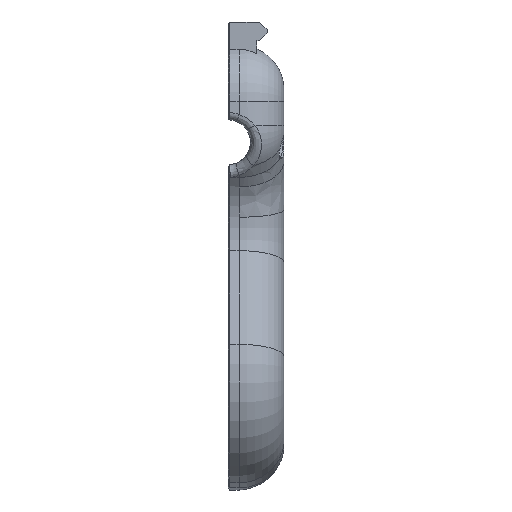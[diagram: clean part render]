
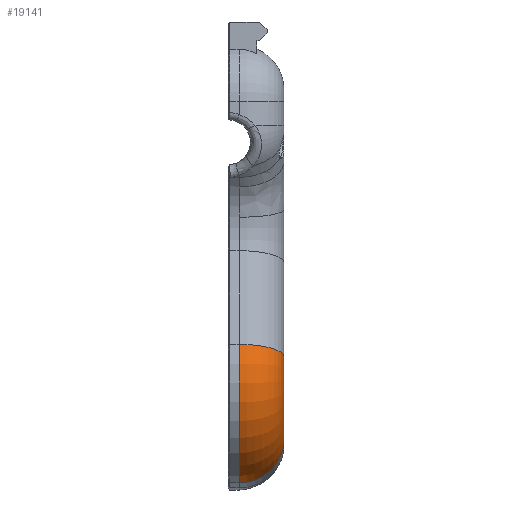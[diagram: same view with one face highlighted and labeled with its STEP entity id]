
A CAD part, left-side view. The second image highlights one B-rep face of the part: STEP entity #19141.
In plain terms, the highlighted toroidal (fillet/blend) face has major radius 18 mm and minor radius 12 mm.
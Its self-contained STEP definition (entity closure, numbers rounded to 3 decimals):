
#64 = PLANE('',#65);
#65 = AXIS2_PLACEMENT_3D('',#66,#67,#68);
#66 = CARTESIAN_POINT('',(10.936,-15.,-32.273));
#67 = DIRECTION('',(0.,-1.,0.));
#68 = DIRECTION('',(0.,0.,-1.));
#674 = VERTEX_POINT('',#675);
#675 = CARTESIAN_POINT('',(-43.196,-15.,-74.47));
#689 = CYLINDRICAL_SURFACE('',#690,12.);
#690 = AXIS2_PLACEMENT_3D('',#691,#692,#693);
#691 = CARTESIAN_POINT('',(-43.196,-3.,-74.47));
#692 = DIRECTION('',(0.276,0.,0.961));
#693 = DIRECTION('',(0.,-1.,0.));
#701 = EDGE_CURVE('',#702,#674,#704,.T.);
#702 = VERTEX_POINT('',#703);
#703 = CARTESIAN_POINT('',(-30.855,-15.,-96.734));
#704 = SURFACE_CURVE('',#705,(#710,#721),.PCURVE_S1.);
#705 = CIRCLE('',#706,18.);
#706 = AXIS2_PLACEMENT_3D('',#707,#708,#709);
#707 = CARTESIAN_POINT('',(-25.893,-15.,-79.431));
#708 = DIRECTION('',(0.,1.,0.));
#709 = DIRECTION('',(-0.276,0.,-0.961));
#710 = PCURVE('',#64,#711);
#711 = DEFINITIONAL_REPRESENTATION('',(#712),#720);
#712 = ( BOUNDED_CURVE() B_SPLINE_CURVE(2,(#713,#714,#715,#716,#717,#718
,#719),.UNSPECIFIED.,.T.,.F.) B_SPLINE_CURVE_WITH_KNOTS((1,2,2,2,2,1),(
    -2.094,0.,2.094,4.189,6.283,
8.378),.UNSPECIFIED.) CURVE() GEOMETRIC_REPRESENTATION_ITEM() 
RATIONAL_B_SPLINE_CURVE((1.,0.5,1.,0.5,1.,0.5,1.)) REPRESENTATION_ITEM(
  '') );
#713 = CARTESIAN_POINT('',(64.461,-41.79));
#714 = CARTESIAN_POINT('',(55.867,-71.759));
#715 = CARTESIAN_POINT('',(34.21,-49.332));
#716 = CARTESIAN_POINT('',(12.553,-26.906));
#717 = CARTESIAN_POINT('',(42.803,-19.363));
#718 = CARTESIAN_POINT('',(73.054,-11.821));
#719 = CARTESIAN_POINT('',(64.461,-41.79));
#720 = ( GEOMETRIC_REPRESENTATION_CONTEXT(2) 
PARAMETRIC_REPRESENTATION_CONTEXT() REPRESENTATION_CONTEXT('2D SPACE',''
  ) );
#721 = PCURVE('',#722,#727);
#722 = TOROIDAL_SURFACE('',#723,18.,12.);
#723 = AXIS2_PLACEMENT_3D('',#724,#725,#726);
#724 = CARTESIAN_POINT('',(-25.893,-3.,-79.431));
#725 = DIRECTION('',(0.,1.,0.));
#726 = DIRECTION('',(-0.276,0.,-0.961));
#727 = DEFINITIONAL_REPRESENTATION('',(#728),#732);
#728 = LINE('',#729,#730);
#729 = CARTESIAN_POINT('',(0.,4.712));
#730 = VECTOR('',#731,1.);
#731 = DIRECTION('',(1.,0.));
#732 = ( GEOMETRIC_REPRESENTATION_CONTEXT(2) 
PARAMETRIC_REPRESENTATION_CONTEXT() REPRESENTATION_CONTEXT('2D SPACE',''
  ) );
#750 = CYLINDRICAL_SURFACE('',#751,12.);
#751 = AXIS2_PLACEMENT_3D('',#752,#753,#754);
#752 = CARTESIAN_POINT('',(-26.048,-3.,-98.112));
#753 = DIRECTION('',(-0.961,0.,0.276));
#754 = DIRECTION('',(0.,-1.,0.));
#19036 = VERTEX_POINT('',#19037);
#19037 = CARTESIAN_POINT('',(-34.162,-3.,-108.269));
#19063 = EDGE_CURVE('',#702,#19036,#19064,.T.);
#19064 = SURFACE_CURVE('',#19065,(#19070,#19076),.PCURVE_S1.);
#19065 = CIRCLE('',#19066,12.);
#19066 = AXIS2_PLACEMENT_3D('',#19067,#19068,#19069);
#19067 = CARTESIAN_POINT('',(-30.855,-3.,-96.734));
#19068 = DIRECTION('',(0.961,0.,-0.276));
#19069 = DIRECTION('',(0.,-1.,0.));
#19070 = PCURVE('',#750,#19071);
#19071 = DEFINITIONAL_REPRESENTATION('',(#19072),#19075);
#19072 = B_SPLINE_CURVE_WITH_KNOTS('',1,(#19073,#19074),.UNSPECIFIED.,
  .F.,.F.,(2,2),(0.,1.571),.PIECEWISE_BEZIER_KNOTS.);
#19073 = CARTESIAN_POINT('',(0.,5.));
#19074 = CARTESIAN_POINT('',(-1.571,5.));
#19075 = ( GEOMETRIC_REPRESENTATION_CONTEXT(2) 
PARAMETRIC_REPRESENTATION_CONTEXT() REPRESENTATION_CONTEXT('2D SPACE',''
  ) );
#19076 = PCURVE('',#722,#19077);
#19077 = DEFINITIONAL_REPRESENTATION('',(#19078),#19081);
#19078 = B_SPLINE_CURVE_WITH_KNOTS('',1,(#19079,#19080),.UNSPECIFIED.,
  .F.,.F.,(2,2),(0.,1.571),.PIECEWISE_BEZIER_KNOTS.);
#19079 = CARTESIAN_POINT('',(0.,4.712));
#19080 = CARTESIAN_POINT('',(0.,6.283));
#19081 = ( GEOMETRIC_REPRESENTATION_CONTEXT(2) 
PARAMETRIC_REPRESENTATION_CONTEXT() REPRESENTATION_CONTEXT('2D SPACE',''
  ) );
#19141 = ADVANCED_FACE('',(#19142),#722,.T.);
#19142 = FACE_BOUND('',#19143,.T.);
#19143 = EDGE_LOOP('',(#19144,#19145,#19146,#19168));
#19144 = ORIENTED_EDGE('',*,*,#19063,.F.);
#19145 = ORIENTED_EDGE('',*,*,#701,.T.);
#19146 = ORIENTED_EDGE('',*,*,#19147,.T.);
#19147 = EDGE_CURVE('',#674,#19148,#19150,.T.);
#19148 = VERTEX_POINT('',#19149);
#19149 = CARTESIAN_POINT('',(-54.731,-3.,-71.162));
#19150 = SURFACE_CURVE('',#19151,(#19156,#19162),.PCURVE_S1.);
#19151 = CIRCLE('',#19152,12.);
#19152 = AXIS2_PLACEMENT_3D('',#19153,#19154,#19155);
#19153 = CARTESIAN_POINT('',(-43.196,-3.,-74.47));
#19154 = DIRECTION('',(-0.276,0.,-0.961));
#19155 = DIRECTION('',(-0.961,0.,0.276));
#19156 = PCURVE('',#722,#19157);
#19157 = DEFINITIONAL_REPRESENTATION('',(#19158),#19161);
#19158 = B_SPLINE_CURVE_WITH_KNOTS('',1,(#19159,#19160),.UNSPECIFIED.,
  .F.,.F.,(2,2),(4.712,6.283),
  .PIECEWISE_BEZIER_KNOTS.);
#19159 = CARTESIAN_POINT('',(1.571,4.712));
#19160 = CARTESIAN_POINT('',(1.571,6.283));
#19161 = ( GEOMETRIC_REPRESENTATION_CONTEXT(2) 
PARAMETRIC_REPRESENTATION_CONTEXT() REPRESENTATION_CONTEXT('2D SPACE',''
  ) );
#19162 = PCURVE('',#689,#19163);
#19163 = DEFINITIONAL_REPRESENTATION('',(#19164),#19167);
#19164 = B_SPLINE_CURVE_WITH_KNOTS('',1,(#19165,#19166),.UNSPECIFIED.,
  .F.,.F.,(2,2),(4.712,6.283),
  .PIECEWISE_BEZIER_KNOTS.);
#19165 = CARTESIAN_POINT('',(0.,0.));
#19166 = CARTESIAN_POINT('',(-1.571,0.));
#19167 = ( GEOMETRIC_REPRESENTATION_CONTEXT(2) 
PARAMETRIC_REPRESENTATION_CONTEXT() REPRESENTATION_CONTEXT('2D SPACE',''
  ) );
#19168 = ORIENTED_EDGE('',*,*,#19169,.F.);
#19169 = EDGE_CURVE('',#19036,#19148,#19170,.T.);
#19170 = SURFACE_CURVE('',#19171,(#19176,#19183),.PCURVE_S1.);
#19171 = CIRCLE('',#19172,30.);
#19172 = AXIS2_PLACEMENT_3D('',#19173,#19174,#19175);
#19173 = CARTESIAN_POINT('',(-25.893,-3.,-79.431));
#19174 = DIRECTION('',(0.,1.,0.));
#19175 = DIRECTION('',(-0.276,0.,-0.961));
#19176 = PCURVE('',#722,#19177);
#19177 = DEFINITIONAL_REPRESENTATION('',(#19178),#19182);
#19178 = LINE('',#19179,#19180);
#19179 = CARTESIAN_POINT('',(0.,6.283));
#19180 = VECTOR('',#19181,1.);
#19181 = DIRECTION('',(1.,0.));
#19182 = ( GEOMETRIC_REPRESENTATION_CONTEXT(2) 
PARAMETRIC_REPRESENTATION_CONTEXT() REPRESENTATION_CONTEXT('2D SPACE',''
  ) );
#19183 = PCURVE('',#19184,#19189);
#19184 = CYLINDRICAL_SURFACE('',#19185,30.);
#19185 = AXIS2_PLACEMENT_3D('',#19186,#19187,#19188);
#19186 = CARTESIAN_POINT('',(-25.893,-15.,-79.431));
#19187 = DIRECTION('',(0.,1.,0.));
#19188 = DIRECTION('',(-0.276,0.,-0.961));
#19189 = DEFINITIONAL_REPRESENTATION('',(#19190),#19194);
#19190 = LINE('',#19191,#19192);
#19191 = CARTESIAN_POINT('',(0.,12.));
#19192 = VECTOR('',#19193,1.);
#19193 = DIRECTION('',(1.,0.));
#19194 = ( GEOMETRIC_REPRESENTATION_CONTEXT(2) 
PARAMETRIC_REPRESENTATION_CONTEXT() REPRESENTATION_CONTEXT('2D SPACE',''
  ) );
